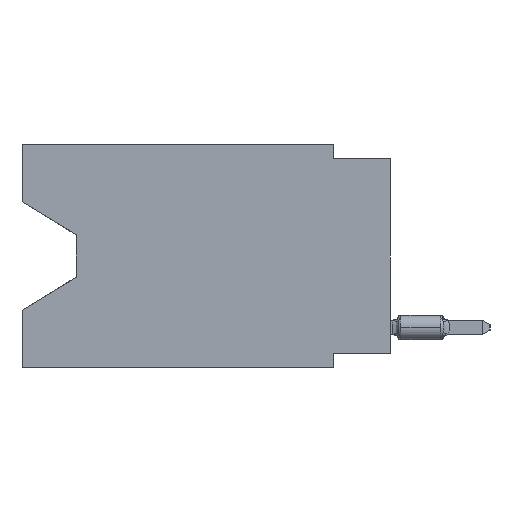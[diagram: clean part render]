
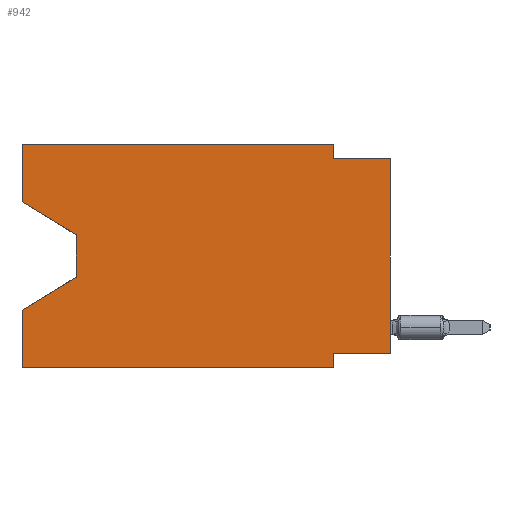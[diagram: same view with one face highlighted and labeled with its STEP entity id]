
A CAD part, left-side view. The second image highlights one B-rep face of the part: STEP entity #942.
In plain terms, the highlighted planar face has unit normal (-1, 0, 0).
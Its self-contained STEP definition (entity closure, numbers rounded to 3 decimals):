
#406 = DIRECTION ( 'NONE',  ( 0., 0., 1. ) ) ;
#942 = ADVANCED_FACE ( 'NONE', ( #18362 ), #13951, .F. ) ;
#1115 = CARTESIAN_POINT ( 'NONE',  ( 0., 2.54, -0.635 ) ) ;
#1434 = EDGE_CURVE ( 'NONE', #13255, #6530, #23544, .T. ) ;
#1824 = EDGE_CURVE ( 'NONE', #13255, #32150, #8144, .T. ) ;
#1848 = ORIENTED_EDGE ( 'NONE', *, *, #27551, .F. ) ;
#1870 = CARTESIAN_POINT ( 'NONE',  ( 0., 16.383, -2.546 ) ) ;
#3100 = DIRECTION ( 'NONE',  ( 0., 0., 1. ) ) ;
#3380 = CARTESIAN_POINT ( 'NONE',  ( 0., 2.54, 0. ) ) ;
#3433 = VECTOR ( 'NONE', #3100, 1000. ) ;
#3486 = ORIENTED_EDGE ( 'NONE', *, *, #15015, .T. ) ;
#3694 = VECTOR ( 'NONE', #25813, 1000. ) ;
#3948 = VECTOR ( 'NONE', #17337, 1000. ) ;
#4613 = VECTOR ( 'NONE', #31570, 1000. ) ;
#5935 = EDGE_CURVE ( 'NONE', #32150, #33342, #18273, .T. ) ;
#6019 = VECTOR ( 'NONE', #7443, 1000. ) ;
#6530 = VERTEX_POINT ( 'NONE', #25244 ) ;
#7025 = CARTESIAN_POINT ( 'NONE',  ( 0., 13.97, -4.013 ) ) ;
#7443 = DIRECTION ( 'NONE',  ( 0., 0., -1. ) ) ;
#7628 = ORIENTED_EDGE ( 'NONE', *, *, #5935, .F. ) ;
#8144 = LINE ( 'NONE', #28718, #4613 ) ;
#8174 = LINE ( 'NONE', #28912, #3433 ) ;
#8621 = EDGE_CURVE ( 'NONE', #12835, #27086, #22067, .T. ) ;
#10056 = EDGE_CURVE ( 'NONE', #31264, #21670, #33045, .T. ) ;
#10366 = CARTESIAN_POINT ( 'NONE',  ( 0., 13.97, -5.893 ) ) ;
#10899 = LINE ( 'NONE', #31455, #21485 ) ;
#12619 = CARTESIAN_POINT ( 'NONE',  ( 0., 2.54, 0. ) ) ;
#12835 = VERTEX_POINT ( 'NONE', #21350 ) ;
#12933 = ORIENTED_EDGE ( 'NONE', *, *, #17094, .F. ) ;
#13109 = DIRECTION ( 'NONE',  ( 0., -1., 0. ) ) ;
#13255 = VERTEX_POINT ( 'NONE', #21311 ) ;
#13530 = LINE ( 'NONE', #31378, #32879 ) ;
#13625 = EDGE_CURVE ( 'NONE', #21670, #30043, #21116, .T. ) ;
#13661 = VERTEX_POINT ( 'NONE', #21434 ) ;
#13692 = DIRECTION ( 'NONE',  ( 0., 0., -1. ) ) ;
#13694 = DIRECTION ( 'NONE',  ( 0., -1., 0. ) ) ;
#13951 = PLANE ( 'NONE',  #20712 ) ;
#14053 = CARTESIAN_POINT ( 'NONE',  ( 0., 16.383, -7.36 ) ) ;
#14786 = VECTOR ( 'NONE', #27520, 1000. ) ;
#15015 = EDGE_CURVE ( 'NONE', #27086, #31692, #33280, .T. ) ;
#15341 = EDGE_CURVE ( 'NONE', #31451, #12835, #27195, .T. ) ;
#16003 = ORIENTED_EDGE ( 'NONE', *, *, #10056, .F. ) ;
#16914 = VECTOR ( 'NONE', #20825, 1000. ) ;
#16966 = ORIENTED_EDGE ( 'NONE', *, *, #13625, .F. ) ;
#17094 = EDGE_CURVE ( 'NONE', #30043, #6530, #10899, .T. ) ;
#17337 = DIRECTION ( 'NONE',  ( 0., 0., -1. ) ) ;
#17531 = CARTESIAN_POINT ( 'NONE',  ( 0., 16.383, 0. ) ) ;
#17946 = EDGE_LOOP ( 'NONE', ( #19875, #30601, #3486, #22033, #28602, #7628, #22908, #22026, #12933, #16966, #16003, #1848 ) ) ;
#18222 = CARTESIAN_POINT ( 'NONE',  ( 0., 16.383, 0. ) ) ;
#18273 = LINE ( 'NONE', #28548, #6019 ) ;
#18362 = FACE_OUTER_BOUND ( 'NONE', #17946, .T. ) ;
#18528 = CARTESIAN_POINT ( 'NONE',  ( 0., 16.383, 0. ) ) ;
#19284 = VECTOR ( 'NONE', #27640, 1000. ) ;
#19875 = ORIENTED_EDGE ( 'NONE', *, *, #15341, .T. ) ;
#20475 = CARTESIAN_POINT ( 'NONE',  ( 0., 13.97, -5.893 ) ) ;
#20577 = LINE ( 'NONE', #17531, #19284 ) ;
#20712 = AXIS2_PLACEMENT_3D ( 'NONE', #18528, #24078, #23922 ) ;
#20825 = DIRECTION ( 'NONE',  ( 0., 0.855, -0.519 ) ) ;
#21116 = LINE ( 'NONE', #3380, #27698 ) ;
#21311 = CARTESIAN_POINT ( 'NONE',  ( 0., 0., -9.271 ) ) ;
#21350 = CARTESIAN_POINT ( 'NONE',  ( 0., 13.97, -4.013 ) ) ;
#21434 = CARTESIAN_POINT ( 'NONE',  ( 0., 16.383, -9.906 ) ) ;
#21485 = VECTOR ( 'NONE', #13109, 1000. ) ;
#21670 = VERTEX_POINT ( 'NONE', #12619 ) ;
#21822 = VECTOR ( 'NONE', #406, 1000. ) ;
#22026 = ORIENTED_EDGE ( 'NONE', *, *, #1434, .T. ) ;
#22033 = ORIENTED_EDGE ( 'NONE', *, *, #29746, .F. ) ;
#22067 = LINE ( 'NONE', #7025, #3948 ) ;
#22505 = EDGE_CURVE ( 'NONE', #13661, #33342, #13530, .T. ) ;
#22908 = ORIENTED_EDGE ( 'NONE', *, *, #1824, .F. ) ;
#23544 = LINE ( 'NONE', #31449, #21822 ) ;
#23922 = DIRECTION ( 'NONE',  ( 0., 0., -1. ) ) ;
#24078 = DIRECTION ( 'NONE',  ( 1., 0., 0. ) ) ;
#25244 = CARTESIAN_POINT ( 'NONE',  ( 0., 0., -0.635 ) ) ;
#25370 = CARTESIAN_POINT ( 'NONE',  ( 0., 16.383, -2.546 ) ) ;
#25813 = DIRECTION ( 'NONE',  ( 0., -1., 0. ) ) ;
#27086 = VERTEX_POINT ( 'NONE', #20475 ) ;
#27195 = LINE ( 'NONE', #1870, #14786 ) ;
#27314 = CARTESIAN_POINT ( 'NONE',  ( 0., 2.54, -9.271 ) ) ;
#27520 = DIRECTION ( 'NONE',  ( 0., -0.855, -0.519 ) ) ;
#27551 = EDGE_CURVE ( 'NONE', #31451, #31264, #8174, .T. ) ;
#27640 = DIRECTION ( 'NONE',  ( 0., 0., 1. ) ) ;
#27698 = VECTOR ( 'NONE', #13692, 1000. ) ;
#28249 = CARTESIAN_POINT ( 'NONE',  ( 0., 16.383, 0. ) ) ;
#28548 = CARTESIAN_POINT ( 'NONE',  ( 0., 2.54, -9.906 ) ) ;
#28602 = ORIENTED_EDGE ( 'NONE', *, *, #22505, .T. ) ;
#28718 = CARTESIAN_POINT ( 'NONE',  ( 0., 0., -9.271 ) ) ;
#28912 = CARTESIAN_POINT ( 'NONE',  ( 0., 16.383, 0. ) ) ;
#29746 = EDGE_CURVE ( 'NONE', #13661, #31692, #20577, .T. ) ;
#30043 = VERTEX_POINT ( 'NONE', #1115 ) ;
#30601 = ORIENTED_EDGE ( 'NONE', *, *, #8621, .T. ) ;
#31264 = VERTEX_POINT ( 'NONE', #28249 ) ;
#31378 = CARTESIAN_POINT ( 'NONE',  ( 0., 16.383, -9.906 ) ) ;
#31449 = CARTESIAN_POINT ( 'NONE',  ( 0., 0., 0. ) ) ;
#31451 = VERTEX_POINT ( 'NONE', #25370 ) ;
#31455 = CARTESIAN_POINT ( 'NONE',  ( 0., 0., -0.635 ) ) ;
#31570 = DIRECTION ( 'NONE',  ( 0., 1., 0. ) ) ;
#31692 = VERTEX_POINT ( 'NONE', #14053 ) ;
#32150 = VERTEX_POINT ( 'NONE', #27314 ) ;
#32692 = CARTESIAN_POINT ( 'NONE',  ( 0., 2.54, -9.906 ) ) ;
#32879 = VECTOR ( 'NONE', #13694, 1000. ) ;
#33045 = LINE ( 'NONE', #18222, #3694 ) ;
#33280 = LINE ( 'NONE', #10366, #16914 ) ;
#33342 = VERTEX_POINT ( 'NONE', #32692 ) ;
